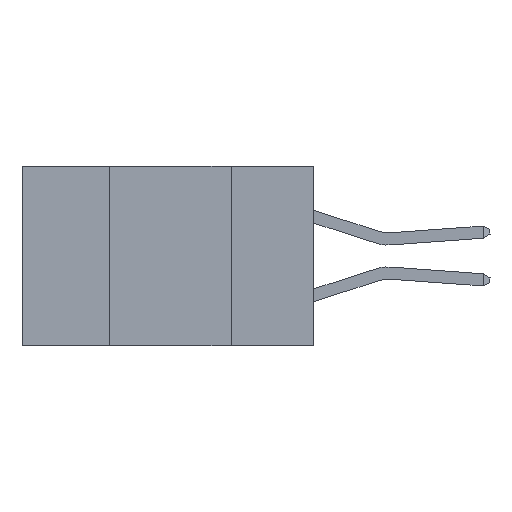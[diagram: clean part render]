
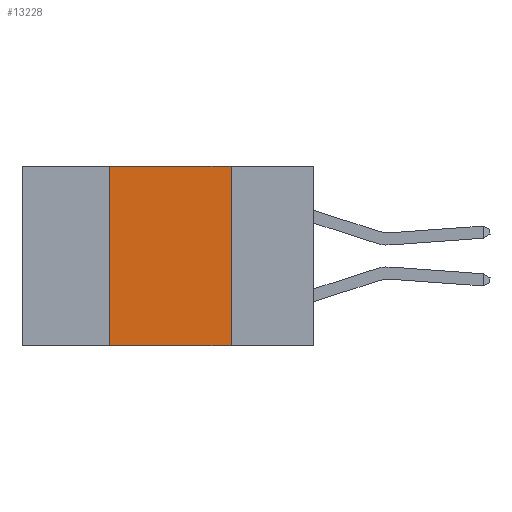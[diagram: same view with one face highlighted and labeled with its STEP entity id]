
A CAD part, left-side view. The second image highlights one B-rep face of the part: STEP entity #13228.
In plain terms, the highlighted planar face has unit normal (-1, 0, 0).
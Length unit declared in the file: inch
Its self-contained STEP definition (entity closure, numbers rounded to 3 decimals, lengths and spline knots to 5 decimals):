
#709 = CARTESIAN_POINT ( 'NONE',  ( 0., 0.17, 0. ) ) ;
#2873 = CARTESIAN_POINT ( 'NONE',  ( 0., 0.17, -0.37 ) ) ;
#3237 = EDGE_CURVE ( 'NONE', #9010, #14641, #19330, .T. ) ;
#3311 = EDGE_CURVE ( 'NONE', #6738, #14641, #3852, .T. ) ;
#3684 = DIRECTION ( 'NONE',  ( 0., 0., -1. ) ) ;
#3852 = LINE ( 'NONE', #20392, #20648 ) ;
#6047 = DIRECTION ( 'NONE',  ( 0., -1., 0. ) ) ;
#6738 = VERTEX_POINT ( 'NONE', #33783 ) ;
#9010 = VERTEX_POINT ( 'NONE', #23602 ) ;
#9328 = EDGE_CURVE ( 'NONE', #6738, #11869, #29386, .T. ) ;
#10080 = DIRECTION ( 'NONE',  ( 0., 0., 1. ) ) ;
#10494 = PLANE ( 'NONE',  #21414 ) ;
#11869 = VERTEX_POINT ( 'NONE', #14294 ) ;
#12659 = CARTESIAN_POINT ( 'NONE',  ( 0., 0.6, 0. ) ) ;
#13128 = EDGE_LOOP ( 'NONE', ( #20182, #28802, #31166, #20424 ) ) ;
#13228 = ADVANCED_FACE ( 'NONE', ( #18175 ), #10494, .F. ) ;
#13278 = DIRECTION ( 'NONE',  ( 0., 0., -1. ) ) ;
#13993 = LINE ( 'NONE', #12659, #35822 ) ;
#14294 = CARTESIAN_POINT ( 'NONE',  ( 0., 0.42, 0. ) ) ;
#14641 = VERTEX_POINT ( 'NONE', #2873 ) ;
#14915 = EDGE_CURVE ( 'NONE', #11869, #9010, #13993, .T. ) ;
#15755 = CARTESIAN_POINT ( 'NONE',  ( 0., 0.6, 0. ) ) ;
#18175 = FACE_OUTER_BOUND ( 'NONE', #13128, .T. ) ;
#19330 = LINE ( 'NONE', #709, #22978 ) ;
#20182 = ORIENTED_EDGE ( 'NONE', *, *, #3237, .F. ) ;
#20392 = CARTESIAN_POINT ( 'NONE',  ( 0., 0.6, -0.37 ) ) ;
#20424 = ORIENTED_EDGE ( 'NONE', *, *, #3311, .T. ) ;
#20648 = VECTOR ( 'NONE', #6047, 39.37008 ) ;
#21414 = AXIS2_PLACEMENT_3D ( 'NONE', #15755, #36575, #13278 ) ;
#21621 = CARTESIAN_POINT ( 'NONE',  ( 0., 0.42, 0. ) ) ;
#22978 = VECTOR ( 'NONE', #3684, 39.37008 ) ;
#23602 = CARTESIAN_POINT ( 'NONE',  ( 0., 0.17, 0. ) ) ;
#27035 = VECTOR ( 'NONE', #10080, 39.37008 ) ;
#28802 = ORIENTED_EDGE ( 'NONE', *, *, #14915, .F. ) ;
#29386 = LINE ( 'NONE', #21621, #27035 ) ;
#31166 = ORIENTED_EDGE ( 'NONE', *, *, #9328, .F. ) ;
#33015 = DIRECTION ( 'NONE',  ( 0., -1., 0. ) ) ;
#33783 = CARTESIAN_POINT ( 'NONE',  ( 0., 0.42, -0.37 ) ) ;
#35822 = VECTOR ( 'NONE', #33015, 39.37008 ) ;
#36575 = DIRECTION ( 'NONE',  ( 1., 0., 0. ) ) ;
